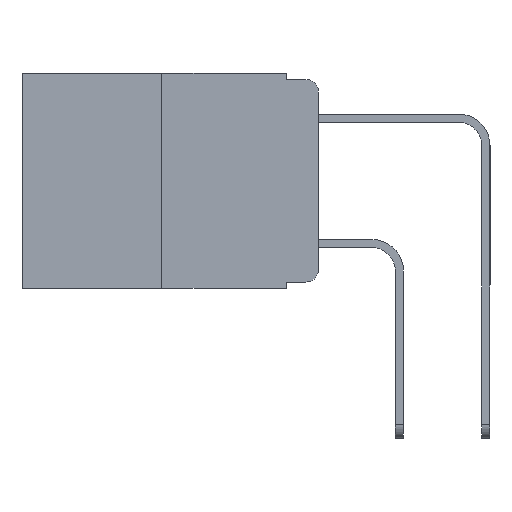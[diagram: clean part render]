
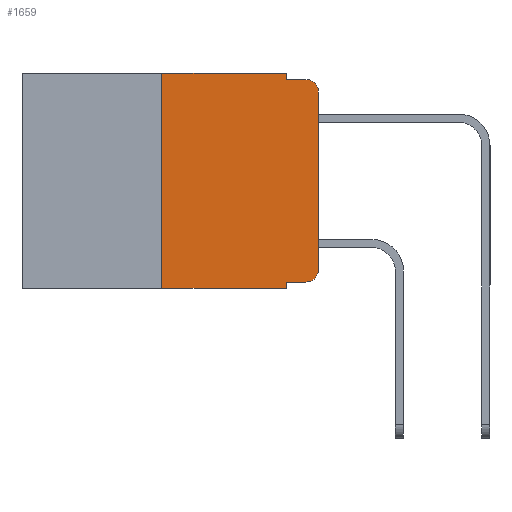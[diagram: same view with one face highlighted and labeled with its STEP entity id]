
A CAD part, left-side view. The second image highlights one B-rep face of the part: STEP entity #1659.
In plain terms, the highlighted planar face has unit normal (-1, 0, 0).
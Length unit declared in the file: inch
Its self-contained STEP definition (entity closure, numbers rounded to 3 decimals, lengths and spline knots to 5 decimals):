
#89 = CARTESIAN_POINT ( 'NONE',  ( 0., 0.051, -0.333 ) ) ;
#145 = VECTOR ( 'NONE', #12633, 39.37008 ) ;
#233 = CARTESIAN_POINT ( 'NONE',  ( 0., 0.051, -0.01 ) ) ;
#514 = CARTESIAN_POINT ( 'NONE',  ( 0., 0., -0.313 ) ) ;
#960 = DIRECTION ( 'NONE',  ( 0., 0., 1. ) ) ;
#1023 = DIRECTION ( 'NONE',  ( -1., 0., 0. ) ) ;
#1123 = CARTESIAN_POINT ( 'NONE',  ( 0., 0.473, -0.343 ) ) ;
#1419 = CARTESIAN_POINT ( 'NONE',  ( 0., 0., -0.03 ) ) ;
#1578 = CARTESIAN_POINT ( 'NONE',  ( 0., 0.02, -0.03 ) ) ;
#1649 = CIRCLE ( 'NONE', #14390, 0.02 ) ;
#1659 = ADVANCED_FACE ( 'NONE', ( #5867 ), #15174, .F. ) ;
#1718 = ORIENTED_EDGE ( 'NONE', *, *, #14820, .T. ) ;
#2138 = VERTEX_POINT ( 'NONE', #3825 ) ;
#2159 = VECTOR ( 'NONE', #11127, 39.37008 ) ;
#2174 = VECTOR ( 'NONE', #16921, 39.37008 ) ;
#2532 = LINE ( 'NONE', #17603, #9598 ) ;
#2892 = VECTOR ( 'NONE', #8590, 39.37008 ) ;
#3045 = EDGE_CURVE ( 'NONE', #11977, #17571, #10780, .T. ) ;
#3065 = DIRECTION ( 'NONE',  ( 0., 0., -1. ) ) ;
#3087 = LINE ( 'NONE', #89, #17292 ) ;
#3303 = ORIENTED_EDGE ( 'NONE', *, *, #8237, .F. ) ;
#3825 = CARTESIAN_POINT ( 'NONE',  ( 0., 0.051, -0.333 ) ) ;
#3919 = VERTEX_POINT ( 'NONE', #13102 ) ;
#3963 = CARTESIAN_POINT ( 'NONE',  ( 0., 0.02, -0.333 ) ) ;
#4359 = VERTEX_POINT ( 'NONE', #7594 ) ;
#4844 = ORIENTED_EDGE ( 'NONE', *, *, #3045, .F. ) ;
#5050 = ORIENTED_EDGE ( 'NONE', *, *, #14396, .T. ) ;
#5146 = VERTEX_POINT ( 'NONE', #1419 ) ;
#5867 = FACE_OUTER_BOUND ( 'NONE', #8960, .T. ) ;
#5997 = LINE ( 'NONE', #16495, #2159 ) ;
#6014 = CARTESIAN_POINT ( 'NONE',  ( 0., 0.051, 0. ) ) ;
#6145 = DIRECTION ( 'NONE',  ( 0., 0., -1. ) ) ;
#6161 = AXIS2_PLACEMENT_3D ( 'NONE', #14464, #6163, #6145 ) ;
#6163 = DIRECTION ( 'NONE',  ( 1., 0., 0. ) ) ;
#6237 = EDGE_CURVE ( 'NONE', #4359, #3919, #2532, .T. ) ;
#6815 = ORIENTED_EDGE ( 'NONE', *, *, #9607, .T. ) ;
#6975 = VERTEX_POINT ( 'NONE', #18133 ) ;
#7166 = LINE ( 'NONE', #15673, #13551 ) ;
#7456 = EDGE_CURVE ( 'NONE', #4359, #6975, #17954, .T. ) ;
#7594 = CARTESIAN_POINT ( 'NONE',  ( 0., 0.25, -0.343 ) ) ;
#8213 = EDGE_CURVE ( 'NONE', #2138, #9122, #3087, .T. ) ;
#8237 = EDGE_CURVE ( 'NONE', #2138, #6975, #16865, .T. ) ;
#8590 = DIRECTION ( 'NONE',  ( 0., -1., 0. ) ) ;
#8679 = EDGE_CURVE ( 'NONE', #17590, #11977, #5997, .T. ) ;
#8960 = EDGE_LOOP ( 'NONE', ( #5050, #6815, #4844, #15568, #10922, #9016, #16842, #3303, #14372, #1718 ) ) ;
#9016 = ORIENTED_EDGE ( 'NONE', *, *, #6237, .F. ) ;
#9122 = VERTEX_POINT ( 'NONE', #3963 ) ;
#9449 = AXIS2_PLACEMENT_3D ( 'NONE', #9578, #1023, #10938 ) ;
#9578 = CARTESIAN_POINT ( 'NONE',  ( 0., 0.02, -0.313 ) ) ;
#9598 = VECTOR ( 'NONE', #960, 39.37008 ) ;
#9607 = EDGE_CURVE ( 'NONE', #5146, #17571, #1649, .T. ) ;
#10151 = DIRECTION ( 'NONE',  ( 0., -1., 0. ) ) ;
#10775 = VECTOR ( 'NONE', #12359, 39.37008 ) ;
#10780 = LINE ( 'NONE', #13980, #2892 ) ;
#10922 = ORIENTED_EDGE ( 'NONE', *, *, #12717, .F. ) ;
#10938 = DIRECTION ( 'NONE',  ( 0., 0., -1. ) ) ;
#11080 = LINE ( 'NONE', #11305, #145 ) ;
#11127 = DIRECTION ( 'NONE',  ( 0., 0., -1. ) ) ;
#11305 = CARTESIAN_POINT ( 'NONE',  ( 0., 0., 0. ) ) ;
#11406 = DIRECTION ( 'NONE',  ( -1., 0., 0. ) ) ;
#11977 = VERTEX_POINT ( 'NONE', #233 ) ;
#12359 = DIRECTION ( 'NONE',  ( 0., -1., 0. ) ) ;
#12633 = DIRECTION ( 'NONE',  ( 0., 0., 1. ) ) ;
#12717 = EDGE_CURVE ( 'NONE', #3919, #17590, #7166, .T. ) ;
#12922 = DIRECTION ( 'NONE',  ( 0., -1., 0. ) ) ;
#13102 = CARTESIAN_POINT ( 'NONE',  ( 0., 0.25, 0. ) ) ;
#13551 = VECTOR ( 'NONE', #12922, 39.37008 ) ;
#13980 = CARTESIAN_POINT ( 'NONE',  ( 0., 0.051, -0.01 ) ) ;
#14372 = ORIENTED_EDGE ( 'NONE', *, *, #8213, .T. ) ;
#14390 = AXIS2_PLACEMENT_3D ( 'NONE', #1578, #11406, #3065 ) ;
#14396 = EDGE_CURVE ( 'NONE', #16624, #5146, #11080, .T. ) ;
#14464 = CARTESIAN_POINT ( 'NONE',  ( 0., 0.473, 0. ) ) ;
#14682 = CIRCLE ( 'NONE', #9449, 0.02 ) ;
#14820 = EDGE_CURVE ( 'NONE', #9122, #16624, #14682, .T. ) ;
#15174 = PLANE ( 'NONE',  #6161 ) ;
#15479 = CARTESIAN_POINT ( 'NONE',  ( 0., 0.02, -0.01 ) ) ;
#15568 = ORIENTED_EDGE ( 'NONE', *, *, #8679, .F. ) ;
#15575 = CARTESIAN_POINT ( 'NONE',  ( 0., 0.051, 0. ) ) ;
#15673 = CARTESIAN_POINT ( 'NONE',  ( 0., 0.473, 0. ) ) ;
#16495 = CARTESIAN_POINT ( 'NONE',  ( 0., 0.051, 0. ) ) ;
#16624 = VERTEX_POINT ( 'NONE', #514 ) ;
#16842 = ORIENTED_EDGE ( 'NONE', *, *, #7456, .T. ) ;
#16865 = LINE ( 'NONE', #15575, #2174 ) ;
#16921 = DIRECTION ( 'NONE',  ( 0., 0., -1. ) ) ;
#17292 = VECTOR ( 'NONE', #10151, 39.37008 ) ;
#17571 = VERTEX_POINT ( 'NONE', #15479 ) ;
#17590 = VERTEX_POINT ( 'NONE', #6014 ) ;
#17603 = CARTESIAN_POINT ( 'NONE',  ( 0., 0.25, 0. ) ) ;
#17954 = LINE ( 'NONE', #1123, #10775 ) ;
#18133 = CARTESIAN_POINT ( 'NONE',  ( 0., 0.051, -0.343 ) ) ;
